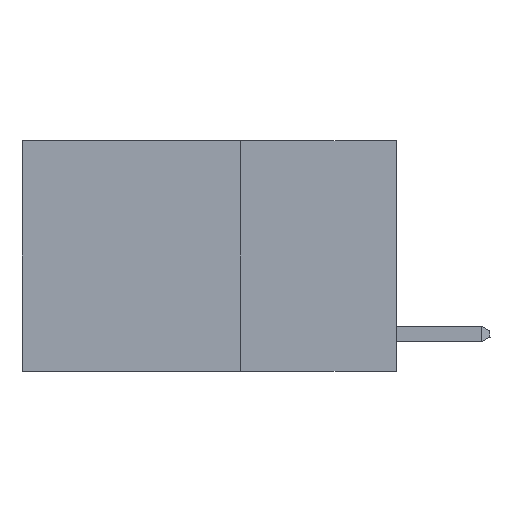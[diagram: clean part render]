
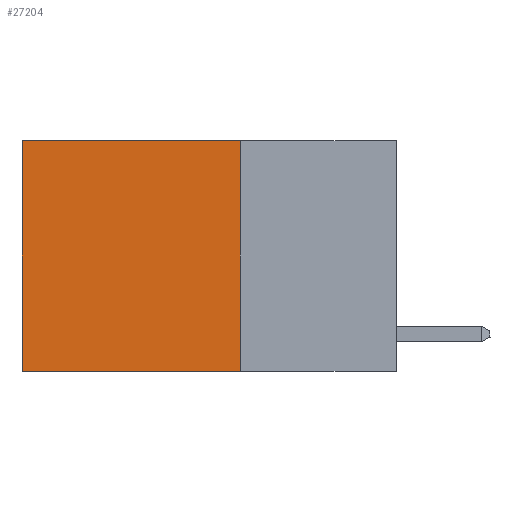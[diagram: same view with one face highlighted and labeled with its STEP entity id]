
A CAD part, left-side view. The second image highlights one B-rep face of the part: STEP entity #27204.
In plain terms, the highlighted planar face has unit normal (-1, 0, 0).
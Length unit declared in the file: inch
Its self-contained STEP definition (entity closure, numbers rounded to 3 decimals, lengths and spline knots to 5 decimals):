
#379 = VERTEX_POINT ( 'NONE', #11766 ) ;
#520 = CARTESIAN_POINT ( 'NONE',  ( 0.2625, 0.25, 0. ) ) ;
#949 = PLANE ( 'NONE',  #23391 ) ;
#3056 = DIRECTION ( 'NONE',  ( 1., 0., 0. ) ) ;
#4666 = VECTOR ( 'NONE', #27931, 39.37008 ) ;
#4873 = DIRECTION ( 'NONE',  ( 0., 0., -1. ) ) ;
#5611 = EDGE_CURVE ( 'NONE', #14988, #379, #21956, .T. ) ;
#6185 = VECTOR ( 'NONE', #4873, 39.37008 ) ;
#6855 = CARTESIAN_POINT ( 'NONE',  ( 0.2625, 0.25, -0.37 ) ) ;
#7134 = LINE ( 'NONE', #15953, #6185 ) ;
#7405 = CARTESIAN_POINT ( 'NONE',  ( 0.2625, 0.25, 0. ) ) ;
#8208 = CARTESIAN_POINT ( 'NONE',  ( 0.2625, 0.25, -0.37 ) ) ;
#11055 = DIRECTION ( 'NONE',  ( 0., 1., 0. ) ) ;
#11766 = CARTESIAN_POINT ( 'NONE',  ( 0.2625, 0.6, 0. ) ) ;
#12291 = ORIENTED_EDGE ( 'NONE', *, *, #18205, .F. ) ;
#12759 = DIRECTION ( 'NONE',  ( 0., 1., 0. ) ) ;
#12791 = LINE ( 'NONE', #19720, #4666 ) ;
#13261 = ORIENTED_EDGE ( 'NONE', *, *, #19430, .F. ) ;
#13463 = CARTESIAN_POINT ( 'NONE',  ( 0.2625, 0.25, 0. ) ) ;
#13834 = FACE_OUTER_BOUND ( 'NONE', #24587, .T. ) ;
#14259 = VERTEX_POINT ( 'NONE', #6855 ) ;
#14327 = ORIENTED_EDGE ( 'NONE', *, *, #5611, .T. ) ;
#14483 = VECTOR ( 'NONE', #11055, 39.37008 ) ;
#14988 = VERTEX_POINT ( 'NONE', #7405 ) ;
#15953 = CARTESIAN_POINT ( 'NONE',  ( 0.2625, 0.25, 0. ) ) ;
#18205 = EDGE_CURVE ( 'NONE', #14259, #20520, #27333, .T. ) ;
#19346 = ORIENTED_EDGE ( 'NONE', *, *, #21134, .T. ) ;
#19430 = EDGE_CURVE ( 'NONE', #14988, #14259, #7134, .T. ) ;
#19720 = CARTESIAN_POINT ( 'NONE',  ( 0.2625, 0.6, 0. ) ) ;
#20520 = VERTEX_POINT ( 'NONE', #23044 ) ;
#21134 = EDGE_CURVE ( 'NONE', #379, #20520, #12791, .T. ) ;
#21956 = LINE ( 'NONE', #13463, #14483 ) ;
#22851 = VECTOR ( 'NONE', #12759, 39.37008 ) ;
#23044 = CARTESIAN_POINT ( 'NONE',  ( 0.2625, 0.6, -0.37 ) ) ;
#23391 = AXIS2_PLACEMENT_3D ( 'NONE', #520, #3056, #24163 ) ;
#24163 = DIRECTION ( 'NONE',  ( 0., 0., -1. ) ) ;
#24587 = EDGE_LOOP ( 'NONE', ( #19346, #12291, #13261, #14327 ) ) ;
#27204 = ADVANCED_FACE ( 'NONE', ( #13834 ), #949, .F. ) ;
#27333 = LINE ( 'NONE', #8208, #22851 ) ;
#27931 = DIRECTION ( 'NONE',  ( 0., 0., -1. ) ) ;
